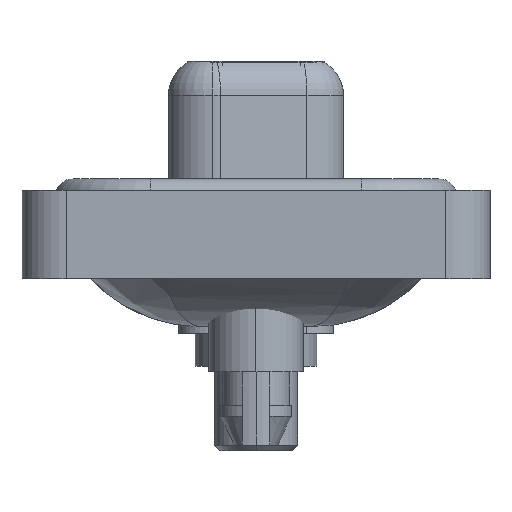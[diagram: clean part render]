
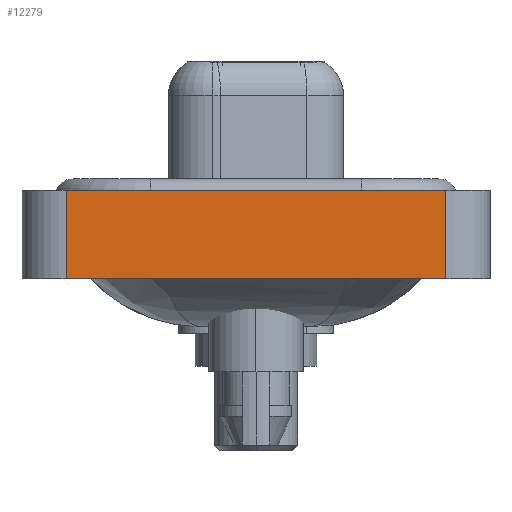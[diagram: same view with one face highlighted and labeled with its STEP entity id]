
A CAD part, left-side view. The second image highlights one B-rep face of the part: STEP entity #12279.
In plain terms, the highlighted planar face has unit normal (-1, 0, 0).
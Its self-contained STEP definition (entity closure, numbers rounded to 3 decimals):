
#26 = DIRECTION ( 'NONE',  ( 0., 0., 1. ) ) ;
#572 = FACE_OUTER_BOUND ( 'NONE', #10581, .T. ) ;
#1347 = LINE ( 'NONE', #6690, #4977 ) ;
#1982 = DIRECTION ( 'NONE',  ( -1., 0., 0. ) ) ;
#2051 = DIRECTION ( 'NONE',  ( 0., -1., 0. ) ) ;
#2133 = CARTESIAN_POINT ( 'NONE',  ( -7.25, -8.55, -3.6 ) ) ;
#2267 = ORIENTED_EDGE ( 'NONE', *, *, #14573, .T. ) ;
#2645 = VECTOR ( 'NONE', #2051, 1000. ) ;
#3123 = PLANE ( 'NONE',  #3960 ) ;
#3960 = AXIS2_PLACEMENT_3D ( 'NONE', #8474, #1982, #7324 ) ;
#4122 = CARTESIAN_POINT ( 'NONE',  ( -7.25, -8.55, -3.6 ) ) ;
#4541 = CARTESIAN_POINT ( 'NONE',  ( -7.25, 8.55, -3.6 ) ) ;
#4583 = VERTEX_POINT ( 'NONE', #8648 ) ;
#4796 = DIRECTION ( 'NONE',  ( 0., 0., 1. ) ) ;
#4977 = VECTOR ( 'NONE', #26, 1000. ) ;
#6690 = CARTESIAN_POINT ( 'NONE',  ( -7.25, -8.55, -3.6 ) ) ;
#6700 = EDGE_CURVE ( 'NONE', #4583, #9003, #8971, .T. ) ;
#7061 = LINE ( 'NONE', #4541, #10179 ) ;
#7324 = DIRECTION ( 'NONE',  ( 0., 0., 1. ) ) ;
#8055 = EDGE_CURVE ( 'NONE', #4583, #11748, #7061, .T. ) ;
#8474 = CARTESIAN_POINT ( 'NONE',  ( -7.25, -8.55, -3.6 ) ) ;
#8648 = CARTESIAN_POINT ( 'NONE',  ( -7.25, 8.55, -3.6 ) ) ;
#8971 = LINE ( 'NONE', #2133, #2645 ) ;
#9003 = VERTEX_POINT ( 'NONE', #4122 ) ;
#9556 = ORIENTED_EDGE ( 'NONE', *, *, #6700, .T. ) ;
#10179 = VECTOR ( 'NONE', #4796, 1000. ) ;
#10581 = EDGE_LOOP ( 'NONE', ( #2267, #15659, #15315, #9556 ) ) ;
#11748 = VERTEX_POINT ( 'NONE', #12151 ) ;
#12151 = CARTESIAN_POINT ( 'NONE',  ( -7.25, 8.55, 0.4 ) ) ;
#12279 = ADVANCED_FACE ( 'NONE', ( #572 ), #3123, .T. ) ;
#13669 = VECTOR ( 'NONE', #15124, 1000. ) ;
#13987 = LINE ( 'NONE', #15389, #13669 ) ;
#14573 = EDGE_CURVE ( 'NONE', #9003, #15179, #1347, .T. ) ;
#15051 = CARTESIAN_POINT ( 'NONE',  ( -7.25, -8.55, 0.4 ) ) ;
#15124 = DIRECTION ( 'NONE',  ( 0., -1., 0. ) ) ;
#15179 = VERTEX_POINT ( 'NONE', #15051 ) ;
#15315 = ORIENTED_EDGE ( 'NONE', *, *, #8055, .F. ) ;
#15389 = CARTESIAN_POINT ( 'NONE',  ( -7.25, -8.55, 0.4 ) ) ;
#15659 = ORIENTED_EDGE ( 'NONE', *, *, #15740, .F. ) ;
#15740 = EDGE_CURVE ( 'NONE', #11748, #15179, #13987, .T. ) ;
